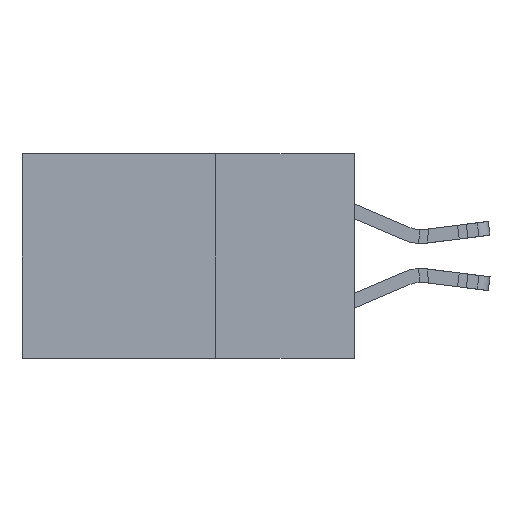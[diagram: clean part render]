
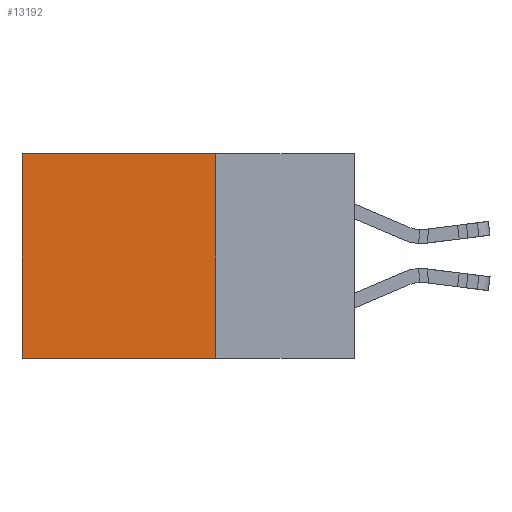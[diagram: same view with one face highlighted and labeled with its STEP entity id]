
A CAD part, left-side view. The second image highlights one B-rep face of the part: STEP entity #13192.
In plain terms, the highlighted planar face has unit normal (-1, 0, 0).
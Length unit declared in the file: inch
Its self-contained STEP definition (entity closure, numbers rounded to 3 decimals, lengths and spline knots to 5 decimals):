
#675 = FACE_OUTER_BOUND ( 'NONE', #13223, .T. ) ;
#1603 = VERTEX_POINT ( 'NONE', #16196 ) ;
#1625 = VECTOR ( 'NONE', #24698, 39.37008 ) ;
#2204 = LINE ( 'NONE', #9450, #1625 ) ;
#2402 = VERTEX_POINT ( 'NONE', #9176 ) ;
#3977 = LINE ( 'NONE', #7902, #24359 ) ;
#4559 = PLANE ( 'NONE',  #12479 ) ;
#5315 = ORIENTED_EDGE ( 'NONE', *, *, #23401, .F. ) ;
#5692 = LINE ( 'NONE', #17972, #15382 ) ;
#6839 = VERTEX_POINT ( 'NONE', #11490 ) ;
#7902 = CARTESIAN_POINT ( 'NONE',  ( 0.2615, 0.25, -0.37 ) ) ;
#8478 = DIRECTION ( 'NONE',  ( 0., 0., -1. ) ) ;
#9176 = CARTESIAN_POINT ( 'NONE',  ( 0.2615, 0.6, -0.37 ) ) ;
#9326 = EDGE_CURVE ( 'NONE', #14571, #6839, #20895, .T. ) ;
#9450 = CARTESIAN_POINT ( 'NONE',  ( 0.2615, 0.25, -0.37 ) ) ;
#10043 = DIRECTION ( 'NONE',  ( 0., 1., 0. ) ) ;
#11490 = CARTESIAN_POINT ( 'NONE',  ( 0.2615, 0.6, 0. ) ) ;
#11789 = CARTESIAN_POINT ( 'NONE',  ( 0.2615, 0.25, 0. ) ) ;
#12479 = AXIS2_PLACEMENT_3D ( 'NONE', #18031, #19891, #8478 ) ;
#13192 = ADVANCED_FACE ( 'NONE', ( #675 ), #4559, .F. ) ;
#13223 = EDGE_LOOP ( 'NONE', ( #22093, #14343, #5315, #20440 ) ) ;
#14343 = ORIENTED_EDGE ( 'NONE', *, *, #21934, .F. ) ;
#14571 = VERTEX_POINT ( 'NONE', #11789 ) ;
#15382 = VECTOR ( 'NONE', #21759, 39.37008 ) ;
#15464 = EDGE_CURVE ( 'NONE', #6839, #2402, #5692, .T. ) ;
#15748 = CARTESIAN_POINT ( 'NONE',  ( 0.2615, 0.25, 0. ) ) ;
#15873 = VECTOR ( 'NONE', #10043, 39.37008 ) ;
#16196 = CARTESIAN_POINT ( 'NONE',  ( 0.2615, 0.25, -0.37 ) ) ;
#17972 = CARTESIAN_POINT ( 'NONE',  ( 0.2615, 0.6, -0.37 ) ) ;
#18031 = CARTESIAN_POINT ( 'NONE',  ( 0.2615, 0.25, -0.37 ) ) ;
#19891 = DIRECTION ( 'NONE',  ( 1., 0., 0. ) ) ;
#20440 = ORIENTED_EDGE ( 'NONE', *, *, #9326, .T. ) ;
#20895 = LINE ( 'NONE', #15748, #15873 ) ;
#21309 = DIRECTION ( 'NONE',  ( 0., 0., -1. ) ) ;
#21759 = DIRECTION ( 'NONE',  ( 0., 0., -1. ) ) ;
#21934 = EDGE_CURVE ( 'NONE', #1603, #2402, #2204, .T. ) ;
#22093 = ORIENTED_EDGE ( 'NONE', *, *, #15464, .T. ) ;
#23401 = EDGE_CURVE ( 'NONE', #14571, #1603, #3977, .T. ) ;
#24359 = VECTOR ( 'NONE', #21309, 39.37008 ) ;
#24698 = DIRECTION ( 'NONE',  ( 0., 1., 0. ) ) ;
